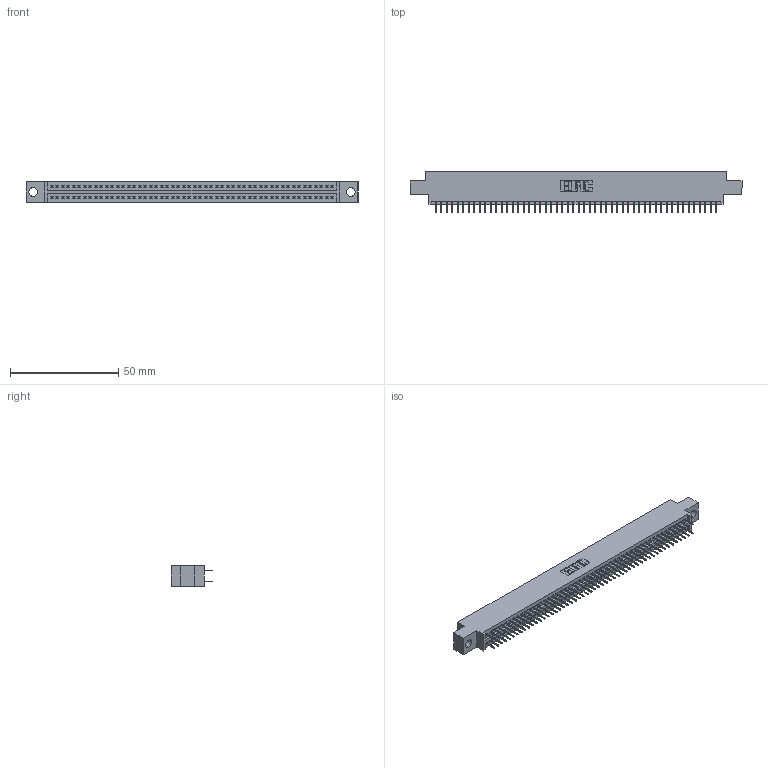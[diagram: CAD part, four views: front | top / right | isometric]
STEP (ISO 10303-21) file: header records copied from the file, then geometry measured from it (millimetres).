
FILE_DESCRIPTION (( 'STEP AP203' ), '1' );
FILE_NAME ('345-104-524-804.STEP', '2021-05-21T13:28:43', ( '' ), ( '' ), 'SwSTEP 2.0', 'SolidWorks 2020', '' );
FILE_SCHEMA (( 'CONFIG_CONTROL_DESIGN' ));
Length unit declared in the file: inch
Products named in the file (3): 345 Part_0.170 Offset - 0.156 Dia-TI; 345-104-524-804; 345-292-001_345-293-124
Assembly tree (105 placements, depth 2):
  345-104-524-804
    345 Part_0.170 Offset - 0.156 Dia-TI
    345-292-001_345-293-124  x104
Bounding box: 153.29 x 19.35 x 9.4 mm (x, y, z)
Volume: 14606.8 mm3; surface area: 21364.5 mm2
Topology: 105 solids, 105 shells, 5760 faces, 16301 edges, 10450 vertices
Faces by surface type: plane 4154, cylinder 1606
Entity records: 40079 total; most frequent: CARTESIAN_POINT 6714, ORIENTED_EDGE 6646, DIRECTION 5907, EDGE_CURVE 3323, LINE 2987, VECTOR 2987, VERTEX_POINT 2210, AXIS2_PLACEMENT_3D 1460
